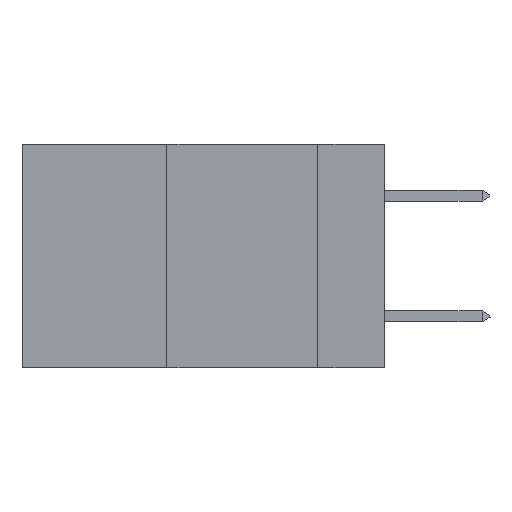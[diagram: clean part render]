
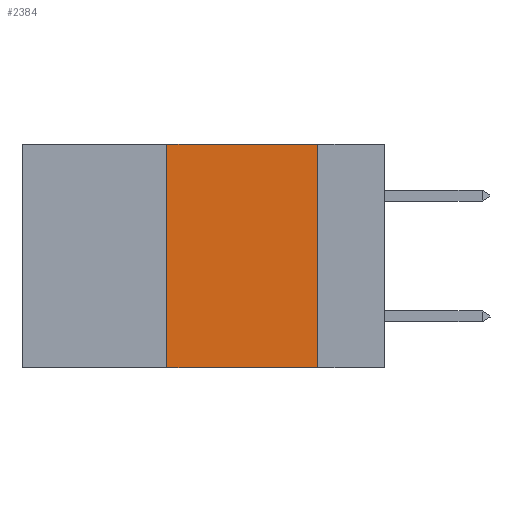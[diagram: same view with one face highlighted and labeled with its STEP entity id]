
A CAD part, left-side view. The second image highlights one B-rep face of the part: STEP entity #2384.
In plain terms, the highlighted planar face has unit normal (-1, 0, 0).
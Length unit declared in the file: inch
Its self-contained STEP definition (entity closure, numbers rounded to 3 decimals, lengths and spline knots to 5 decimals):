
#512 = CARTESIAN_POINT ( 'NONE',  ( 0., 0.6, -0.37 ) ) ;
#975 = EDGE_CURVE ( 'NONE', #4110, #10413, #2119, .T. ) ;
#2086 = LINE ( 'NONE', #16328, #11574 ) ;
#2119 = LINE ( 'NONE', #512, #21769 ) ;
#2169 = AXIS2_PLACEMENT_3D ( 'NONE', #8709, #18169, #6791 ) ;
#2384 = ADVANCED_FACE ( 'NONE', ( #17170 ), #20340, .F. ) ;
#3136 = ORIENTED_EDGE ( 'NONE', *, *, #11040, .F. ) ;
#3334 = EDGE_LOOP ( 'NONE', ( #10580, #3136, #17338, #19862 ) ) ;
#3840 = DIRECTION ( 'NONE',  ( 0., 0., 1. ) ) ;
#4110 = VERTEX_POINT ( 'NONE', #10165 ) ;
#4941 = DIRECTION ( 'NONE',  ( 0., 0., -1. ) ) ;
#5231 = EDGE_CURVE ( 'NONE', #16100, #10413, #2086, .T. ) ;
#5833 = VECTOR ( 'NONE', #13754, 39.37008 ) ;
#6202 = DIRECTION ( 'NONE',  ( 0., -1., 0. ) ) ;
#6791 = DIRECTION ( 'NONE',  ( 0., 0., -1. ) ) ;
#8331 = VERTEX_POINT ( 'NONE', #20611 ) ;
#8549 = LINE ( 'NONE', #16048, #5833 ) ;
#8709 = CARTESIAN_POINT ( 'NONE',  ( 0., 0.6, 0. ) ) ;
#10165 = CARTESIAN_POINT ( 'NONE',  ( 0., 0.36, -0.37 ) ) ;
#10413 = VERTEX_POINT ( 'NONE', #15253 ) ;
#10580 = ORIENTED_EDGE ( 'NONE', *, *, #5231, .F. ) ;
#11040 = EDGE_CURVE ( 'NONE', #8331, #16100, #8549, .T. ) ;
#11371 = LINE ( 'NONE', #13472, #20890 ) ;
#11574 = VECTOR ( 'NONE', #4941, 39.37008 ) ;
#13472 = CARTESIAN_POINT ( 'NONE',  ( 0., 0.36, 0. ) ) ;
#13754 = DIRECTION ( 'NONE',  ( 0., -1., 0. ) ) ;
#15253 = CARTESIAN_POINT ( 'NONE',  ( 0., 0.11, -0.37 ) ) ;
#16048 = CARTESIAN_POINT ( 'NONE',  ( 0., 0.6, 0. ) ) ;
#16100 = VERTEX_POINT ( 'NONE', #20708 ) ;
#16328 = CARTESIAN_POINT ( 'NONE',  ( 0., 0.11, 0. ) ) ;
#17170 = FACE_OUTER_BOUND ( 'NONE', #3334, .T. ) ;
#17338 = ORIENTED_EDGE ( 'NONE', *, *, #20182, .F. ) ;
#18169 = DIRECTION ( 'NONE',  ( 1., 0., 0. ) ) ;
#19862 = ORIENTED_EDGE ( 'NONE', *, *, #975, .T. ) ;
#20182 = EDGE_CURVE ( 'NONE', #4110, #8331, #11371, .T. ) ;
#20340 = PLANE ( 'NONE',  #2169 ) ;
#20611 = CARTESIAN_POINT ( 'NONE',  ( 0., 0.36, 0. ) ) ;
#20708 = CARTESIAN_POINT ( 'NONE',  ( 0., 0.11, 0. ) ) ;
#20890 = VECTOR ( 'NONE', #3840, 39.37008 ) ;
#21769 = VECTOR ( 'NONE', #6202, 39.37008 ) ;
